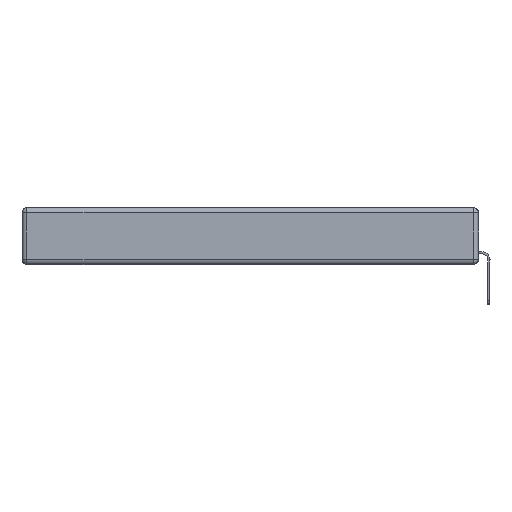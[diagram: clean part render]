
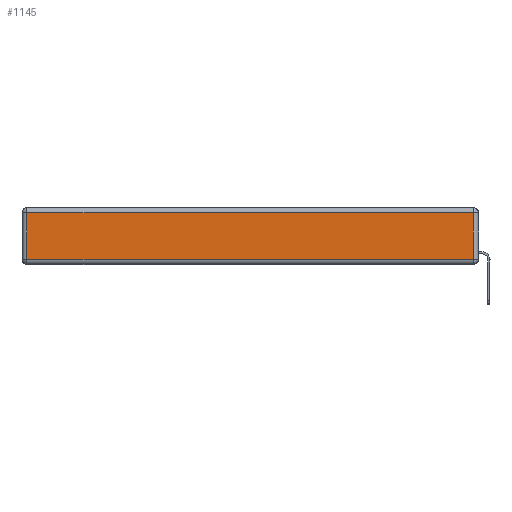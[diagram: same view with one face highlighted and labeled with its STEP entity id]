
A CAD part, left-side view. The second image highlights one B-rep face of the part: STEP entity #1145.
In plain terms, the highlighted planar face has unit normal (-1, 0, 0).
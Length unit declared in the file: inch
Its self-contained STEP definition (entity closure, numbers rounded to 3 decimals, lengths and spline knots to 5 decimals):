
#183 = LINE ( 'NONE', #21469, #20933 ) ;
#416 = CARTESIAN_POINT ( 'NONE',  ( 0., 2.72, -0.313 ) ) ;
#1145 = ADVANCED_FACE ( 'NONE', ( #19254 ), #1566, .T. ) ;
#1566 = PLANE ( 'NONE',  #6972 ) ;
#1827 = LINE ( 'NONE', #19285, #8926 ) ;
#2046 = DIRECTION ( 'NONE',  ( 0., 1., 0. ) ) ;
#2430 = ORIENTED_EDGE ( 'NONE', *, *, #4180, .T. ) ;
#3516 = DIRECTION ( 'NONE',  ( -1., 0., 0. ) ) ;
#4152 = VERTEX_POINT ( 'NONE', #416 ) ;
#4180 = EDGE_CURVE ( 'NONE', #22142, #20246, #183, .T. ) ;
#4521 = EDGE_CURVE ( 'NONE', #6173, #22142, #20657, .T. ) ;
#5111 = DIRECTION ( 'NONE',  ( 0., 0., 1. ) ) ;
#5261 = DIRECTION ( 'NONE',  ( 0., -1., 0. ) ) ;
#5568 = ORIENTED_EDGE ( 'NONE', *, *, #4521, .T. ) ;
#6173 = VERTEX_POINT ( 'NONE', #11816 ) ;
#6356 = EDGE_CURVE ( 'NONE', #20246, #4152, #14480, .T. ) ;
#6841 = CARTESIAN_POINT ( 'NONE',  ( 0., 0.03, -0.343 ) ) ;
#6972 = AXIS2_PLACEMENT_3D ( 'NONE', #21098, #3516, #5111 ) ;
#7210 = DIRECTION ( 'NONE',  ( 0., 0., -1. ) ) ;
#8926 = VECTOR ( 'NONE', #5261, 39.37008 ) ;
#9090 = CARTESIAN_POINT ( 'NONE',  ( 0., 2.72, -0.03 ) ) ;
#11816 = CARTESIAN_POINT ( 'NONE',  ( 0., 0.03, -0.313 ) ) ;
#13825 = VECTOR ( 'NONE', #7210, 39.37008 ) ;
#14480 = LINE ( 'NONE', #21138, #13825 ) ;
#15367 = EDGE_CURVE ( 'NONE', #4152, #6173, #1827, .T. ) ;
#16361 = EDGE_LOOP ( 'NONE', ( #21845, #5568, #2430, #21165 ) ) ;
#17437 = DIRECTION ( 'NONE',  ( 0., 0., 1. ) ) ;
#18587 = CARTESIAN_POINT ( 'NONE',  ( 0., 0.03, -0.03 ) ) ;
#19254 = FACE_OUTER_BOUND ( 'NONE', #16361, .T. ) ;
#19285 = CARTESIAN_POINT ( 'NONE',  ( 0., 0., -0.313 ) ) ;
#20246 = VERTEX_POINT ( 'NONE', #9090 ) ;
#20657 = LINE ( 'NONE', #6841, #22439 ) ;
#20933 = VECTOR ( 'NONE', #2046, 39.37008 ) ;
#21098 = CARTESIAN_POINT ( 'NONE',  ( 0., 0., -0.343 ) ) ;
#21138 = CARTESIAN_POINT ( 'NONE',  ( 0., 2.72, -0.343 ) ) ;
#21165 = ORIENTED_EDGE ( 'NONE', *, *, #6356, .T. ) ;
#21469 = CARTESIAN_POINT ( 'NONE',  ( 0., 2.75, -0.03 ) ) ;
#21845 = ORIENTED_EDGE ( 'NONE', *, *, #15367, .T. ) ;
#22142 = VERTEX_POINT ( 'NONE', #18587 ) ;
#22439 = VECTOR ( 'NONE', #17437, 39.37008 ) ;
